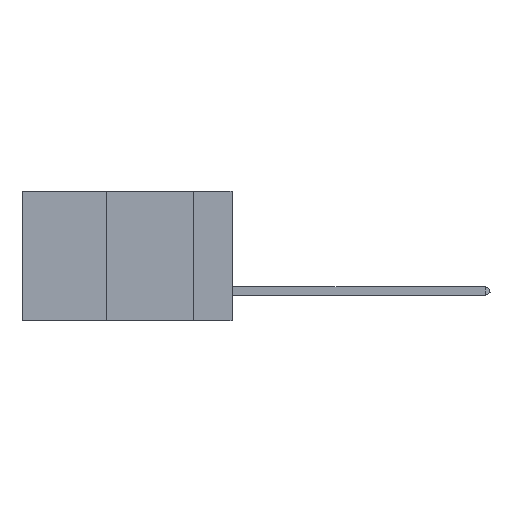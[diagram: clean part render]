
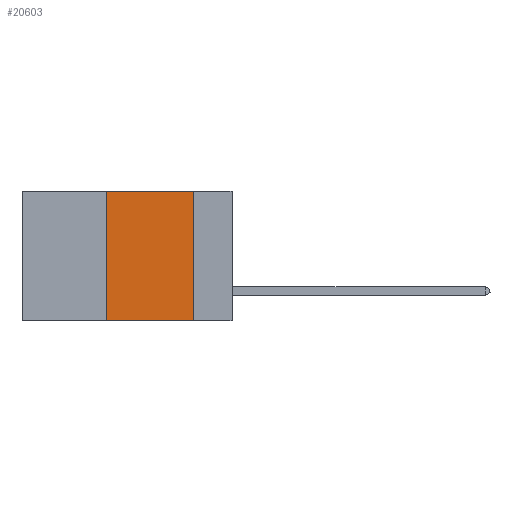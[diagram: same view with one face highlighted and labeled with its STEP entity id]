
A CAD part, left-side view. The second image highlights one B-rep face of the part: STEP entity #20603.
In plain terms, the highlighted planar face has unit normal (-1, 0, 0).
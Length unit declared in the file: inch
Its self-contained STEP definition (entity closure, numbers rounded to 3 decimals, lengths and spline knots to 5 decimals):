
#785 = CARTESIAN_POINT ( 'NONE',  ( 0., 0.6, 0. ) ) ;
#3430 = ORIENTED_EDGE ( 'NONE', *, *, #20211, .F. ) ;
#3840 = EDGE_CURVE ( 'NONE', #8030, #45657, #25867, .T. ) ;
#3941 = LINE ( 'NONE', #33043, #33530 ) ;
#4606 = VECTOR ( 'NONE', #9420, 39.37008 ) ;
#4658 = EDGE_CURVE ( 'NONE', #25806, #32264, #35404, .T. ) ;
#4947 = CARTESIAN_POINT ( 'NONE',  ( 0., 0.36, -0.37 ) ) ;
#5886 = EDGE_LOOP ( 'NONE', ( #41825, #33915, #3430, #23878 ) ) ;
#6777 = LINE ( 'NONE', #23761, #8576 ) ;
#8030 = VERTEX_POINT ( 'NONE', #40023 ) ;
#8576 = VECTOR ( 'NONE', #42502, 39.37008 ) ;
#8695 = CARTESIAN_POINT ( 'NONE',  ( 0., 0.6, 0. ) ) ;
#9420 = DIRECTION ( 'NONE',  ( 0., -1., 0. ) ) ;
#12910 = DIRECTION ( 'NONE',  ( 0., -1., 0. ) ) ;
#16603 = DIRECTION ( 'NONE',  ( 1., 0., 0. ) ) ;
#20211 = EDGE_CURVE ( 'NONE', #25806, #8030, #3941, .T. ) ;
#20603 = ADVANCED_FACE ( 'NONE', ( #42567 ), #23922, .F. ) ;
#20888 = CARTESIAN_POINT ( 'NONE',  ( 0., 0.11, -0.37 ) ) ;
#21531 = CARTESIAN_POINT ( 'NONE',  ( 0., 0.6, -0.37 ) ) ;
#23761 = CARTESIAN_POINT ( 'NONE',  ( 0., 0.11, 0. ) ) ;
#23878 = ORIENTED_EDGE ( 'NONE', *, *, #4658, .T. ) ;
#23922 = PLANE ( 'NONE',  #34276 ) ;
#24600 = CARTESIAN_POINT ( 'NONE',  ( 0., 0.11, 0. ) ) ;
#25806 = VERTEX_POINT ( 'NONE', #4947 ) ;
#25867 = LINE ( 'NONE', #785, #27652 ) ;
#27652 = VECTOR ( 'NONE', #12910, 39.37008 ) ;
#32017 = DIRECTION ( 'NONE',  ( 0., 0., -1. ) ) ;
#32264 = VERTEX_POINT ( 'NONE', #20888 ) ;
#32596 = EDGE_CURVE ( 'NONE', #45657, #32264, #6777, .T. ) ;
#33043 = CARTESIAN_POINT ( 'NONE',  ( 0., 0.36, 0. ) ) ;
#33530 = VECTOR ( 'NONE', #48567, 39.37008 ) ;
#33915 = ORIENTED_EDGE ( 'NONE', *, *, #3840, .F. ) ;
#34276 = AXIS2_PLACEMENT_3D ( 'NONE', #8695, #16603, #32017 ) ;
#35404 = LINE ( 'NONE', #21531, #4606 ) ;
#40023 = CARTESIAN_POINT ( 'NONE',  ( 0., 0.36, 0. ) ) ;
#41825 = ORIENTED_EDGE ( 'NONE', *, *, #32596, .F. ) ;
#42502 = DIRECTION ( 'NONE',  ( 0., 0., -1. ) ) ;
#42567 = FACE_OUTER_BOUND ( 'NONE', #5886, .T. ) ;
#45657 = VERTEX_POINT ( 'NONE', #24600 ) ;
#48567 = DIRECTION ( 'NONE',  ( 0., 0., 1. ) ) ;
